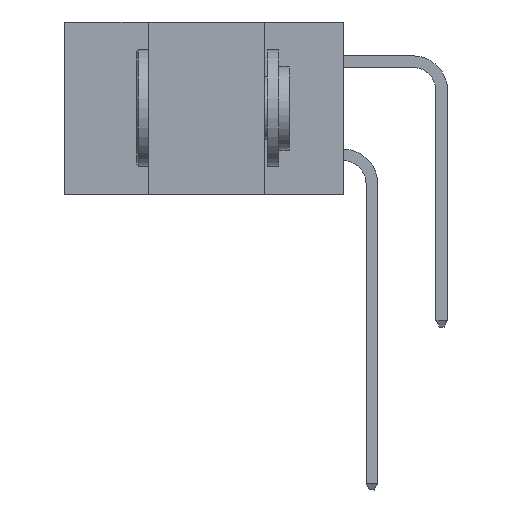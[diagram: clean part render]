
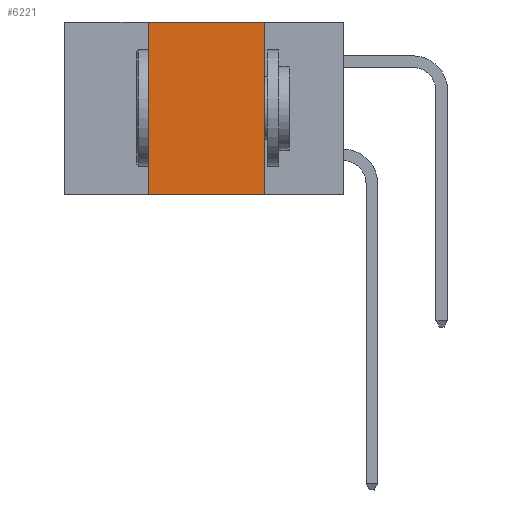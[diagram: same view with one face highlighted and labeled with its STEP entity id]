
A CAD part, left-side view. The second image highlights one B-rep face of the part: STEP entity #6221.
In plain terms, the highlighted planar face has unit normal (-1, 0, 0).
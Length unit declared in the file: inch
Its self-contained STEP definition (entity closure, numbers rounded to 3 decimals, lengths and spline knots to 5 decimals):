
#234 = PLANE ( 'NONE',  #1360 ) ;
#772 = LINE ( 'NONE', #5974, #9688 ) ;
#997 = CARTESIAN_POINT ( 'NONE',  ( 0., 0.6, 0. ) ) ;
#1284 = EDGE_CURVE ( 'NONE', #9336, #6660, #3587, .T. ) ;
#1360 = AXIS2_PLACEMENT_3D ( 'NONE', #10788, #15945, #13160 ) ;
#1458 = DIRECTION ( 'NONE',  ( 0., -1., 0. ) ) ;
#1592 = FACE_OUTER_BOUND ( 'NONE', #10652, .T. ) ;
#2163 = ORIENTED_EDGE ( 'NONE', *, *, #1284, .F. ) ;
#3408 = CARTESIAN_POINT ( 'NONE',  ( 0., 0.42, 0. ) ) ;
#3498 = CARTESIAN_POINT ( 'NONE',  ( 0., 0.42, -0.37 ) ) ;
#3541 = VERTEX_POINT ( 'NONE', #8167 ) ;
#3587 = LINE ( 'NONE', #3498, #12211 ) ;
#3788 = ORIENTED_EDGE ( 'NONE', *, *, #5997, .F. ) ;
#4161 = EDGE_CURVE ( 'NONE', #3541, #4713, #772, .T. ) ;
#4211 = ORIENTED_EDGE ( 'NONE', *, *, #4161, .F. ) ;
#4713 = VERTEX_POINT ( 'NONE', #6254 ) ;
#5094 = DIRECTION ( 'NONE',  ( 0., -1., 0. ) ) ;
#5974 = CARTESIAN_POINT ( 'NONE',  ( 0., 0.17, -0.37 ) ) ;
#5997 = EDGE_CURVE ( 'NONE', #6660, #3541, #16623, .T. ) ;
#6221 = ADVANCED_FACE ( 'NONE', ( #1592 ), #234, .F. ) ;
#6254 = CARTESIAN_POINT ( 'NONE',  ( 0., 0.17, -0.37 ) ) ;
#6307 = DIRECTION ( 'NONE',  ( 0., 0., 1. ) ) ;
#6660 = VERTEX_POINT ( 'NONE', #3408 ) ;
#6738 = LINE ( 'NONE', #13201, #13179 ) ;
#7796 = ORIENTED_EDGE ( 'NONE', *, *, #8049, .T. ) ;
#8049 = EDGE_CURVE ( 'NONE', #9336, #4713, #6738, .T. ) ;
#8167 = CARTESIAN_POINT ( 'NONE',  ( 0., 0.17, 0. ) ) ;
#9336 = VERTEX_POINT ( 'NONE', #11268 ) ;
#9688 = VECTOR ( 'NONE', #15046, 39.37008 ) ;
#10652 = EDGE_LOOP ( 'NONE', ( #4211, #3788, #2163, #7796 ) ) ;
#10788 = CARTESIAN_POINT ( 'NONE',  ( 0., 0.6, 0. ) ) ;
#11268 = CARTESIAN_POINT ( 'NONE',  ( 0., 0.42, -0.37 ) ) ;
#12211 = VECTOR ( 'NONE', #6307, 39.37008 ) ;
#13160 = DIRECTION ( 'NONE',  ( 0., 0., -1. ) ) ;
#13179 = VECTOR ( 'NONE', #1458, 39.37008 ) ;
#13201 = CARTESIAN_POINT ( 'NONE',  ( 0., 0.6, -0.37 ) ) ;
#15046 = DIRECTION ( 'NONE',  ( 0., 0., -1. ) ) ;
#15640 = VECTOR ( 'NONE', #5094, 39.37008 ) ;
#15945 = DIRECTION ( 'NONE',  ( 1., 0., 0. ) ) ;
#16623 = LINE ( 'NONE', #997, #15640 ) ;
